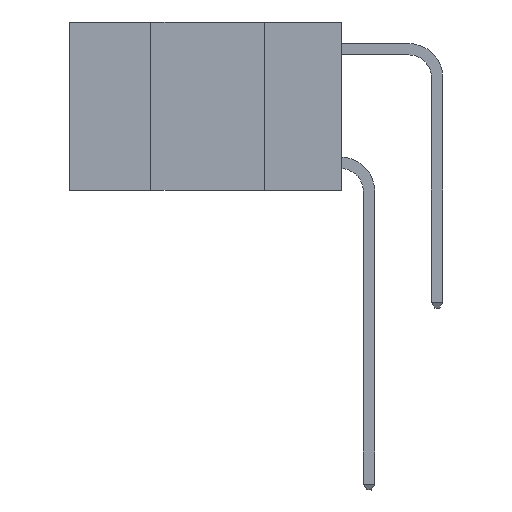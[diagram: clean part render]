
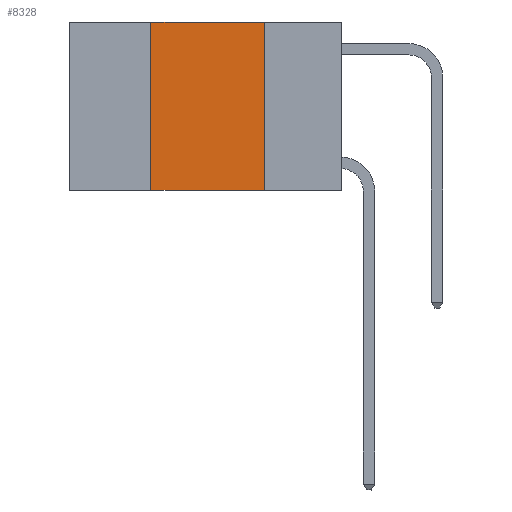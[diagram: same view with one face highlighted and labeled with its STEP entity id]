
A CAD part, left-side view. The second image highlights one B-rep face of the part: STEP entity #8328.
In plain terms, the highlighted planar face has unit normal (-1, 0, 0).
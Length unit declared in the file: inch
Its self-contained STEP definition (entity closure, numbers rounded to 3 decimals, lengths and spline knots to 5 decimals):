
#496 = CARTESIAN_POINT ( 'NONE',  ( 0., 0.42, 0. ) ) ;
#830 = ORIENTED_EDGE ( 'NONE', *, *, #4985, .T. ) ;
#893 = EDGE_CURVE ( 'NONE', #9837, #9699, #7713, .T. ) ;
#1042 = CARTESIAN_POINT ( 'NONE',  ( 0., 0.42, -0.37 ) ) ;
#1331 = CARTESIAN_POINT ( 'NONE',  ( 0., 0.42, 0. ) ) ;
#1576 = EDGE_LOOP ( 'NONE', ( #2179, #8192, #2671, #830 ) ) ;
#1607 = DIRECTION ( 'NONE',  ( 0., -1., 0. ) ) ;
#2045 = VECTOR ( 'NONE', #7409, 39.37008 ) ;
#2179 = ORIENTED_EDGE ( 'NONE', *, *, #2538, .F. ) ;
#2538 = EDGE_CURVE ( 'NONE', #9699, #8677, #10480, .T. ) ;
#2671 = ORIENTED_EDGE ( 'NONE', *, *, #8902, .F. ) ;
#3525 = FACE_OUTER_BOUND ( 'NONE', #1576, .T. ) ;
#4985 = EDGE_CURVE ( 'NONE', #10869, #8677, #10847, .T. ) ;
#5002 = CARTESIAN_POINT ( 'NONE',  ( 0., 0.6, -0.37 ) ) ;
#5417 = CARTESIAN_POINT ( 'NONE',  ( 0., 0.17, 0. ) ) ;
#5516 = VECTOR ( 'NONE', #7050, 39.37008 ) ;
#5829 = DIRECTION ( 'NONE',  ( 0., 0., -1. ) ) ;
#6977 = AXIS2_PLACEMENT_3D ( 'NONE', #9933, #10873, #5829 ) ;
#7050 = DIRECTION ( 'NONE',  ( 0., -1., 0. ) ) ;
#7392 = CARTESIAN_POINT ( 'NONE',  ( 0., 0.6, 0. ) ) ;
#7409 = DIRECTION ( 'NONE',  ( 0., 0., 1. ) ) ;
#7476 = DIRECTION ( 'NONE',  ( 0., 0., -1. ) ) ;
#7653 = CARTESIAN_POINT ( 'NONE',  ( 0., 0.17, 0. ) ) ;
#7713 = LINE ( 'NONE', #7392, #5516 ) ;
#7939 = CARTESIAN_POINT ( 'NONE',  ( 0., 0.17, -0.37 ) ) ;
#8192 = ORIENTED_EDGE ( 'NONE', *, *, #893, .F. ) ;
#8198 = VECTOR ( 'NONE', #7476, 39.37008 ) ;
#8289 = VECTOR ( 'NONE', #1607, 39.37008 ) ;
#8328 = ADVANCED_FACE ( 'NONE', ( #3525 ), #9970, .F. ) ;
#8677 = VERTEX_POINT ( 'NONE', #7939 ) ;
#8902 = EDGE_CURVE ( 'NONE', #10869, #9837, #9272, .T. ) ;
#9272 = LINE ( 'NONE', #496, #2045 ) ;
#9699 = VERTEX_POINT ( 'NONE', #5417 ) ;
#9837 = VERTEX_POINT ( 'NONE', #1331 ) ;
#9933 = CARTESIAN_POINT ( 'NONE',  ( 0., 0.6, 0. ) ) ;
#9970 = PLANE ( 'NONE',  #6977 ) ;
#10480 = LINE ( 'NONE', #7653, #8198 ) ;
#10847 = LINE ( 'NONE', #5002, #8289 ) ;
#10869 = VERTEX_POINT ( 'NONE', #1042 ) ;
#10873 = DIRECTION ( 'NONE',  ( 1., 0., 0. ) ) ;
